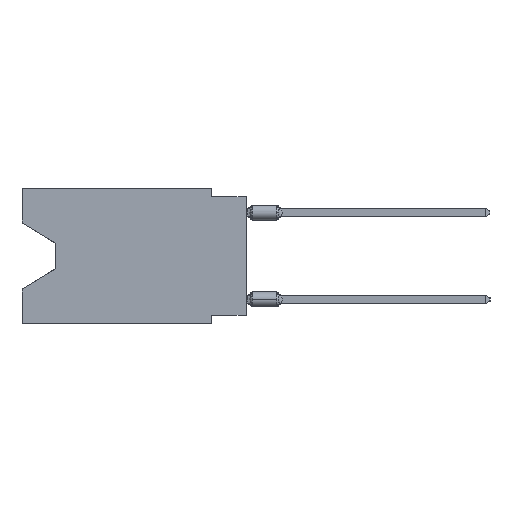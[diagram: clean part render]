
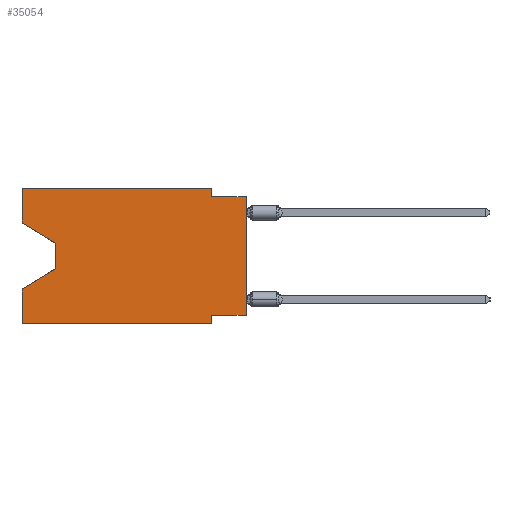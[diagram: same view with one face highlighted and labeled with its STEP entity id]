
A CAD part, left-side view. The second image highlights one B-rep face of the part: STEP entity #35054.
In plain terms, the highlighted planar face has unit normal (-1, 0, 0).
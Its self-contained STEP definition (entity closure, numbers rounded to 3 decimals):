
#325 = CARTESIAN_POINT ( 'NONE',  ( 0., 16.383, 0. ) ) ;
#354 = CARTESIAN_POINT ( 'NONE',  ( 0., 16.383, -2.546 ) ) ;
#1032 = CARTESIAN_POINT ( 'NONE',  ( 0., 0., -0.635 ) ) ;
#1799 = CARTESIAN_POINT ( 'NONE',  ( 0., 16.383, -9.906 ) ) ;
#3197 = CARTESIAN_POINT ( 'NONE',  ( 0., 16.383, 0. ) ) ;
#3280 = CARTESIAN_POINT ( 'NONE',  ( 0., 2.54, -9.271 ) ) ;
#4585 = ORIENTED_EDGE ( 'NONE', *, *, #23007, .F. ) ;
#4906 = ORIENTED_EDGE ( 'NONE', *, *, #44040, .F. ) ;
#5149 = ORIENTED_EDGE ( 'NONE', *, *, #29599, .F. ) ;
#5604 = DIRECTION ( 'NONE',  ( 0., 0., -1. ) ) ;
#5612 = CARTESIAN_POINT ( 'NONE',  ( 0., 0., 0. ) ) ;
#5806 = ORIENTED_EDGE ( 'NONE', *, *, #8752, .T. ) ;
#6406 = VECTOR ( 'NONE', #21419, 1000. ) ;
#6708 = EDGE_CURVE ( 'NONE', #42320, #19915, #20153, .T. ) ;
#7704 = LINE ( 'NONE', #22161, #29142 ) ;
#7816 = LINE ( 'NONE', #61155, #49085 ) ;
#8074 = VERTEX_POINT ( 'NONE', #45327 ) ;
#8161 = VERTEX_POINT ( 'NONE', #51560 ) ;
#8752 = EDGE_CURVE ( 'NONE', #9305, #56797, #39502, .T. ) ;
#9187 = DIRECTION ( 'NONE',  ( 0., 0., -1. ) ) ;
#9305 = VERTEX_POINT ( 'NONE', #21502 ) ;
#9508 = VECTOR ( 'NONE', #53952, 1000. ) ;
#10653 = EDGE_LOOP ( 'NONE', ( #39083, #15480, #30730, #51242, #5806, #51929, #21549, #23855, #4585, #5149, #4906, #18711 ) ) ;
#10671 = LINE ( 'NONE', #325, #48365 ) ;
#11796 = DIRECTION ( 'NONE',  ( 0., -1., 0. ) ) ;
#11847 = DIRECTION ( 'NONE',  ( 0., -1., 0. ) ) ;
#15480 = ORIENTED_EDGE ( 'NONE', *, *, #54969, .T. ) ;
#15756 = EDGE_CURVE ( 'NONE', #9305, #42363, #7816, .T. ) ;
#16173 = CARTESIAN_POINT ( 'NONE',  ( 0., 13.97, -5.893 ) ) ;
#16690 = LINE ( 'NONE', #1032, #6406 ) ;
#17638 = DIRECTION ( 'NONE',  ( 0., 0.855, -0.519 ) ) ;
#18470 = VERTEX_POINT ( 'NONE', #16173 ) ;
#18711 = ORIENTED_EDGE ( 'NONE', *, *, #20521, .F. ) ;
#19190 = DIRECTION ( 'NONE',  ( 0., -0.855, -0.519 ) ) ;
#19915 = VERTEX_POINT ( 'NONE', #3280 ) ;
#20153 = LINE ( 'NONE', #58428, #54994 ) ;
#20296 = LINE ( 'NONE', #53865, #52543 ) ;
#20382 = VERTEX_POINT ( 'NONE', #47754 ) ;
#20521 = EDGE_CURVE ( 'NONE', #33376, #53338, #10671, .T. ) ;
#21040 = CARTESIAN_POINT ( 'NONE',  ( 0., 0., -9.271 ) ) ;
#21419 = DIRECTION ( 'NONE',  ( 0., -1., 0. ) ) ;
#21502 = CARTESIAN_POINT ( 'NONE',  ( 0., 16.383, -9.906 ) ) ;
#21549 = ORIENTED_EDGE ( 'NONE', *, *, #6708, .F. ) ;
#21670 = DIRECTION ( 'NONE',  ( 0., 0., -1. ) ) ;
#22161 = CARTESIAN_POINT ( 'NONE',  ( 0., 2.54, 0. ) ) ;
#23007 = EDGE_CURVE ( 'NONE', #20382, #32321, #16690, .T. ) ;
#23855 = ORIENTED_EDGE ( 'NONE', *, *, #55371, .T. ) ;
#23874 = DIRECTION ( 'NONE',  ( 0., 0., 1. ) ) ;
#26385 = LINE ( 'NONE', #49929, #60577 ) ;
#26665 = DIRECTION ( 'NONE',  ( 0., 0., 1. ) ) ;
#28091 = CARTESIAN_POINT ( 'NONE',  ( 0., 2.54, -9.906 ) ) ;
#28861 = PLANE ( 'NONE',  #60624 ) ;
#29142 = VECTOR ( 'NONE', #59820, 1000. ) ;
#29599 = EDGE_CURVE ( 'NONE', #8074, #20382, #7704, .T. ) ;
#30062 = VECTOR ( 'NONE', #11847, 1000. ) ;
#30730 = ORIENTED_EDGE ( 'NONE', *, *, #33226, .T. ) ;
#32321 = VERTEX_POINT ( 'NONE', #50440 ) ;
#33226 = EDGE_CURVE ( 'NONE', #18470, #42363, #35261, .T. ) ;
#33376 = VERTEX_POINT ( 'NONE', #57790 ) ;
#33434 = EDGE_CURVE ( 'NONE', #33376, #8161, #58099, .T. ) ;
#35054 = ADVANCED_FACE ( 'NONE', ( #43302 ), #28861, .F. ) ;
#35261 = LINE ( 'NONE', #41500, #36415 ) ;
#36415 = VECTOR ( 'NONE', #17638, 1000. ) ;
#39083 = ORIENTED_EDGE ( 'NONE', *, *, #33434, .T. ) ;
#39502 = LINE ( 'NONE', #1799, #30062 ) ;
#39837 = LINE ( 'NONE', #5612, #9508 ) ;
#40506 = CARTESIAN_POINT ( 'NONE',  ( 0., 16.383, -7.36 ) ) ;
#41500 = CARTESIAN_POINT ( 'NONE',  ( 0., 13.97, -5.893 ) ) ;
#42320 = VERTEX_POINT ( 'NONE', #21040 ) ;
#42363 = VERTEX_POINT ( 'NONE', #40506 ) ;
#43302 = FACE_OUTER_BOUND ( 'NONE', #10653, .T. ) ;
#43446 = VECTOR ( 'NONE', #19190, 1000. ) ;
#43726 = CARTESIAN_POINT ( 'NONE',  ( 0., 2.54, -9.906 ) ) ;
#43969 = VECTOR ( 'NONE', #9187, 1000. ) ;
#44040 = EDGE_CURVE ( 'NONE', #53338, #8074, #20296, .T. ) ;
#45327 = CARTESIAN_POINT ( 'NONE',  ( 0., 2.54, 0. ) ) ;
#47356 = EDGE_CURVE ( 'NONE', #19915, #56797, #52191, .T. ) ;
#47754 = CARTESIAN_POINT ( 'NONE',  ( 0., 2.54, -0.635 ) ) ;
#48000 = CARTESIAN_POINT ( 'NONE',  ( 0., 16.383, 0. ) ) ;
#48365 = VECTOR ( 'NONE', #23874, 1000. ) ;
#49085 = VECTOR ( 'NONE', #26665, 1000. ) ;
#49929 = CARTESIAN_POINT ( 'NONE',  ( 0., 13.97, -4.013 ) ) ;
#50440 = CARTESIAN_POINT ( 'NONE',  ( 0., 0., -0.635 ) ) ;
#51242 = ORIENTED_EDGE ( 'NONE', *, *, #15756, .F. ) ;
#51560 = CARTESIAN_POINT ( 'NONE',  ( 0., 13.97, -4.013 ) ) ;
#51929 = ORIENTED_EDGE ( 'NONE', *, *, #47356, .F. ) ;
#52191 = LINE ( 'NONE', #43726, #43969 ) ;
#52543 = VECTOR ( 'NONE', #11796, 1000. ) ;
#53020 = DIRECTION ( 'NONE',  ( 1., 0., 0. ) ) ;
#53338 = VERTEX_POINT ( 'NONE', #3197 ) ;
#53726 = DIRECTION ( 'NONE',  ( 0., 1., 0. ) ) ;
#53865 = CARTESIAN_POINT ( 'NONE',  ( 0., 16.383, 0. ) ) ;
#53952 = DIRECTION ( 'NONE',  ( 0., 0., 1. ) ) ;
#54969 = EDGE_CURVE ( 'NONE', #8161, #18470, #26385, .T. ) ;
#54994 = VECTOR ( 'NONE', #53726, 1000. ) ;
#55371 = EDGE_CURVE ( 'NONE', #42320, #32321, #39837, .T. ) ;
#56797 = VERTEX_POINT ( 'NONE', #28091 ) ;
#57790 = CARTESIAN_POINT ( 'NONE',  ( 0., 16.383, -2.546 ) ) ;
#58099 = LINE ( 'NONE', #354, #43446 ) ;
#58428 = CARTESIAN_POINT ( 'NONE',  ( 0., 0., -9.271 ) ) ;
#59820 = DIRECTION ( 'NONE',  ( 0., 0., -1. ) ) ;
#60577 = VECTOR ( 'NONE', #21670, 1000. ) ;
#60624 = AXIS2_PLACEMENT_3D ( 'NONE', #48000, #53020, #5604 ) ;
#61155 = CARTESIAN_POINT ( 'NONE',  ( 0., 16.383, 0. ) ) ;
